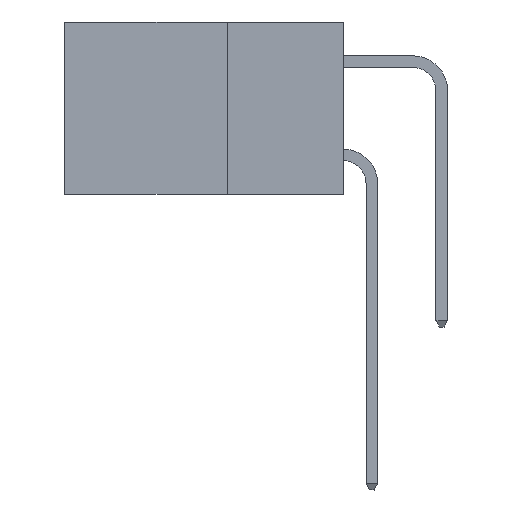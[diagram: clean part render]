
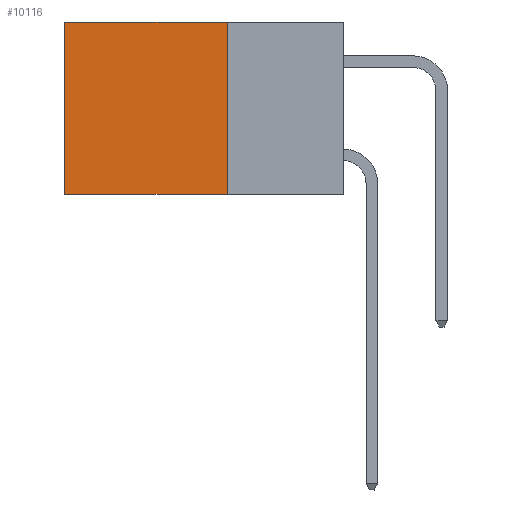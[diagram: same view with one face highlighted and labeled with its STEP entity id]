
A CAD part, left-side view. The second image highlights one B-rep face of the part: STEP entity #10116.
In plain terms, the highlighted planar face has unit normal (-1, 0, 0).
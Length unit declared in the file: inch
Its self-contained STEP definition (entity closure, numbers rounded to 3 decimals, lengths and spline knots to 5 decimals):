
#736 = VERTEX_POINT ( 'NONE', #5207 ) ;
#752 = DIRECTION ( 'NONE',  ( 0., 0., -1. ) ) ;
#999 = EDGE_CURVE ( 'NONE', #736, #10744, #7422, .T. ) ;
#1424 = DIRECTION ( 'NONE',  ( 0., 0., -1. ) ) ;
#2094 = EDGE_CURVE ( 'NONE', #14183, #10257, #9428, .T. ) ;
#2133 = CARTESIAN_POINT ( 'NONE',  ( 0.2615, 0.25, -0.37 ) ) ;
#2877 = ORIENTED_EDGE ( 'NONE', *, *, #999, .F. ) ;
#3562 = ORIENTED_EDGE ( 'NONE', *, *, #6637, .T. ) ;
#3879 = VECTOR ( 'NONE', #1424, 39.37008 ) ;
#4466 = ORIENTED_EDGE ( 'NONE', *, *, #2094, .T. ) ;
#5190 = CARTESIAN_POINT ( 'NONE',  ( 0.2615, 0.25, 0. ) ) ;
#5207 = CARTESIAN_POINT ( 'NONE',  ( 0.2615, 0.25, 0. ) ) ;
#5795 = VECTOR ( 'NONE', #752, 39.37008 ) ;
#6084 = VECTOR ( 'NONE', #8707, 39.37008 ) ;
#6348 = DIRECTION ( 'NONE',  ( 1., 0., 0. ) ) ;
#6637 = EDGE_CURVE ( 'NONE', #736, #14183, #13068, .T. ) ;
#6702 = CARTESIAN_POINT ( 'NONE',  ( 0.2615, 0.6, -0.37 ) ) ;
#7422 = LINE ( 'NONE', #11876, #5795 ) ;
#7693 = EDGE_LOOP ( 'NONE', ( #4466, #9370, #2877, #3562 ) ) ;
#8036 = CARTESIAN_POINT ( 'NONE',  ( 0.2615, 0.6, -0.37 ) ) ;
#8707 = DIRECTION ( 'NONE',  ( 0., 1., 0. ) ) ;
#9370 = ORIENTED_EDGE ( 'NONE', *, *, #10398, .F. ) ;
#9428 = LINE ( 'NONE', #8036, #3879 ) ;
#9662 = DIRECTION ( 'NONE',  ( 0., 1., 0. ) ) ;
#9801 = LINE ( 'NONE', #14220, #6084 ) ;
#10116 = ADVANCED_FACE ( 'NONE', ( #12840 ), #13861, .F. ) ;
#10257 = VERTEX_POINT ( 'NONE', #6702 ) ;
#10398 = EDGE_CURVE ( 'NONE', #10744, #10257, #9801, .T. ) ;
#10744 = VERTEX_POINT ( 'NONE', #2133 ) ;
#11168 = VECTOR ( 'NONE', #9662, 39.37008 ) ;
#11481 = CARTESIAN_POINT ( 'NONE',  ( 0.2615, 0.6, 0. ) ) ;
#11876 = CARTESIAN_POINT ( 'NONE',  ( 0.2615, 0.25, -0.37 ) ) ;
#12840 = FACE_OUTER_BOUND ( 'NONE', #7693, .T. ) ;
#13068 = LINE ( 'NONE', #5190, #11168 ) ;
#13099 = AXIS2_PLACEMENT_3D ( 'NONE', #13990, #6348, #13923 ) ;
#13861 = PLANE ( 'NONE',  #13099 ) ;
#13923 = DIRECTION ( 'NONE',  ( 0., 0., -1. ) ) ;
#13990 = CARTESIAN_POINT ( 'NONE',  ( 0.2615, 0.25, -0.37 ) ) ;
#14183 = VERTEX_POINT ( 'NONE', #11481 ) ;
#14220 = CARTESIAN_POINT ( 'NONE',  ( 0.2615, 0.25, -0.37 ) ) ;
